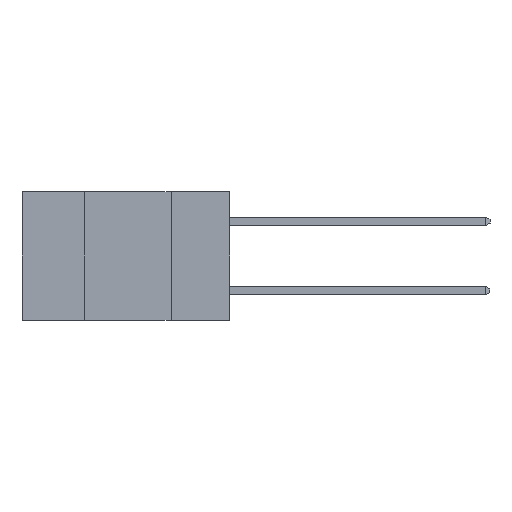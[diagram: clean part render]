
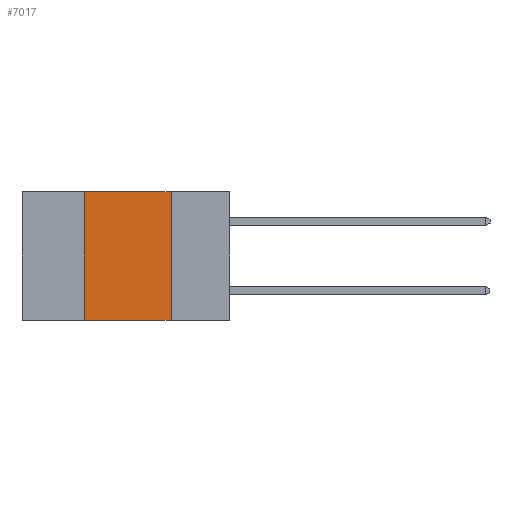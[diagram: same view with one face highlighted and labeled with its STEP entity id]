
A CAD part, left-side view. The second image highlights one B-rep face of the part: STEP entity #7017.
In plain terms, the highlighted planar face has unit normal (-1, 0, 0).
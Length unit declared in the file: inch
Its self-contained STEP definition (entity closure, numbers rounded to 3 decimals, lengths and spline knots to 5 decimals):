
#31 = CARTESIAN_POINT ( 'NONE',  ( 0., 0.17, 0. ) ) ;
#491 = VECTOR ( 'NONE', #4607, 39.37008 ) ;
#601 = DIRECTION ( 'NONE',  ( 0., 0., 1. ) ) ;
#910 = AXIS2_PLACEMENT_3D ( 'NONE', #2486, #8447, #3409 ) ;
#1839 = LINE ( 'NONE', #8441, #10233 ) ;
#2061 = CARTESIAN_POINT ( 'NONE',  ( 0., 0.42, -0.37 ) ) ;
#2260 = VERTEX_POINT ( 'NONE', #2061 ) ;
#2486 = CARTESIAN_POINT ( 'NONE',  ( 0., 0.6, 0. ) ) ;
#2540 = VERTEX_POINT ( 'NONE', #4830 ) ;
#3056 = VERTEX_POINT ( 'NONE', #7418 ) ;
#3201 = LINE ( 'NONE', #31, #491 ) ;
#3238 = VECTOR ( 'NONE', #6466, 39.37008 ) ;
#3401 = DIRECTION ( 'NONE',  ( 0., -1., 0. ) ) ;
#3409 = DIRECTION ( 'NONE',  ( 0., 0., -1. ) ) ;
#3528 = LINE ( 'NONE', #10049, #3238 ) ;
#4607 = DIRECTION ( 'NONE',  ( 0., 0., -1. ) ) ;
#4830 = CARTESIAN_POINT ( 'NONE',  ( 0., 0.17, -0.37 ) ) ;
#5231 = EDGE_CURVE ( 'NONE', #2260, #2540, #3528, .T. ) ;
#5442 = EDGE_CURVE ( 'NONE', #3056, #8521, #1839, .T. ) ;
#5622 = FACE_OUTER_BOUND ( 'NONE', #9005, .T. ) ;
#5663 = VECTOR ( 'NONE', #601, 39.37008 ) ;
#5842 = EDGE_CURVE ( 'NONE', #2260, #3056, #5942, .T. ) ;
#5942 = LINE ( 'NONE', #8377, #5663 ) ;
#6466 = DIRECTION ( 'NONE',  ( 0., -1., 0. ) ) ;
#6614 = ORIENTED_EDGE ( 'NONE', *, *, #5842, .F. ) ;
#6752 = EDGE_CURVE ( 'NONE', #8521, #2540, #3201, .T. ) ;
#7017 = ADVANCED_FACE ( 'NONE', ( #5622 ), #10492, .F. ) ;
#7418 = CARTESIAN_POINT ( 'NONE',  ( 0., 0.42, 0. ) ) ;
#7482 = CARTESIAN_POINT ( 'NONE',  ( 0., 0.17, 0. ) ) ;
#8187 = ORIENTED_EDGE ( 'NONE', *, *, #5442, .F. ) ;
#8377 = CARTESIAN_POINT ( 'NONE',  ( 0., 0.42, 0. ) ) ;
#8441 = CARTESIAN_POINT ( 'NONE',  ( 0., 0.6, 0. ) ) ;
#8447 = DIRECTION ( 'NONE',  ( 1., 0., 0. ) ) ;
#8521 = VERTEX_POINT ( 'NONE', #7482 ) ;
#8614 = ORIENTED_EDGE ( 'NONE', *, *, #5231, .T. ) ;
#9005 = EDGE_LOOP ( 'NONE', ( #9771, #8187, #6614, #8614 ) ) ;
#9771 = ORIENTED_EDGE ( 'NONE', *, *, #6752, .F. ) ;
#10049 = CARTESIAN_POINT ( 'NONE',  ( 0., 0.6, -0.37 ) ) ;
#10233 = VECTOR ( 'NONE', #3401, 39.37008 ) ;
#10492 = PLANE ( 'NONE',  #910 ) ;
